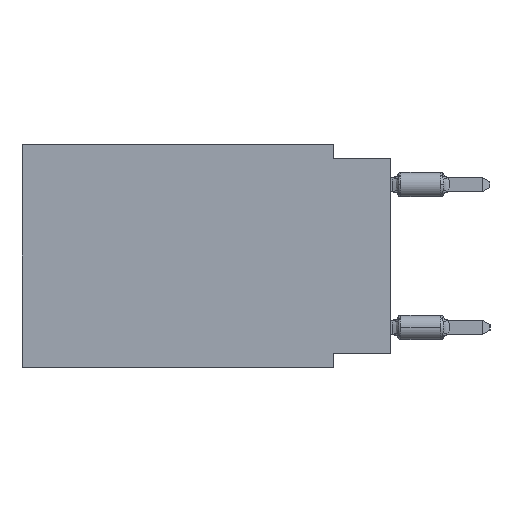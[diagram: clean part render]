
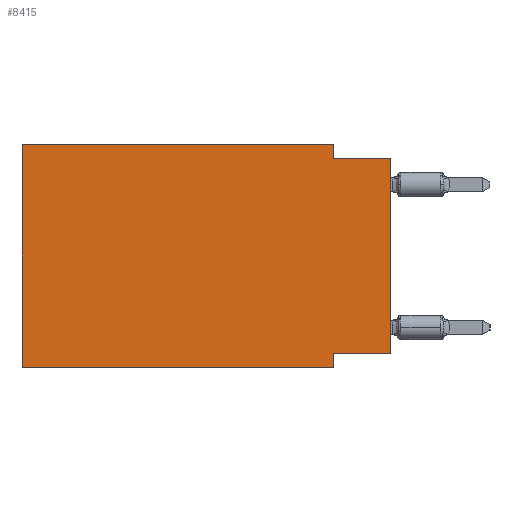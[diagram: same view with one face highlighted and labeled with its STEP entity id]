
A CAD part, left-side view. The second image highlights one B-rep face of the part: STEP entity #8415.
In plain terms, the highlighted planar face has unit normal (-1, 0, 0).
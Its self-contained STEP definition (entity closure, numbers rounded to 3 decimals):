
#71 = VECTOR ( 'NONE', #8384, 1000. ) ;
#573 = ORIENTED_EDGE ( 'NONE', *, *, #8297, .F. ) ;
#647 = VECTOR ( 'NONE', #6000, 1000. ) ;
#902 = VERTEX_POINT ( 'NONE', #19983 ) ;
#1110 = AXIS2_PLACEMENT_3D ( 'NONE', #20146, #5331, #11951 ) ;
#1647 = VERTEX_POINT ( 'NONE', #11638 ) ;
#1866 = CARTESIAN_POINT ( 'NONE',  ( 0., 2.54, -9.906 ) ) ;
#2638 = LINE ( 'NONE', #6296, #17011 ) ;
#3402 = PLANE ( 'NONE',  #1110 ) ;
#4509 = VERTEX_POINT ( 'NONE', #14054 ) ;
#4520 = LINE ( 'NONE', #7998, #15049 ) ;
#4533 = LINE ( 'NONE', #14067, #17102 ) ;
#5331 = DIRECTION ( 'NONE',  ( 1., 0., 0. ) ) ;
#5632 = VERTEX_POINT ( 'NONE', #18513 ) ;
#5681 = CARTESIAN_POINT ( 'NONE',  ( 0., 0., -0.635 ) ) ;
#5980 = DIRECTION ( 'NONE',  ( 0., 0., 1. ) ) ;
#6000 = DIRECTION ( 'NONE',  ( 0., 0., 1. ) ) ;
#6167 = CARTESIAN_POINT ( 'NONE',  ( 0., 2.54, 0. ) ) ;
#6296 = CARTESIAN_POINT ( 'NONE',  ( 0., 2.54, 0. ) ) ;
#6753 = FACE_OUTER_BOUND ( 'NONE', #12081, .T. ) ;
#7368 = DIRECTION ( 'NONE',  ( 0., -1., 0. ) ) ;
#7404 = ORIENTED_EDGE ( 'NONE', *, *, #13579, .F. ) ;
#7580 = DIRECTION ( 'NONE',  ( 0., -1., 0. ) ) ;
#7770 = VECTOR ( 'NONE', #7368, 1000. ) ;
#7865 = LINE ( 'NONE', #11325, #647 ) ;
#7998 = CARTESIAN_POINT ( 'NONE',  ( 0., 0., -9.271 ) ) ;
#8297 = EDGE_CURVE ( 'NONE', #1647, #11531, #18009, .T. ) ;
#8384 = DIRECTION ( 'NONE',  ( 0., -1., 0. ) ) ;
#8415 = ADVANCED_FACE ( 'NONE', ( #6753 ), #3402, .F. ) ;
#8666 = ORIENTED_EDGE ( 'NONE', *, *, #11497, .T. ) ;
#8861 = ORIENTED_EDGE ( 'NONE', *, *, #14319, .F. ) ;
#9248 = DIRECTION ( 'NONE',  ( 0., 0., -1. ) ) ;
#9490 = LINE ( 'NONE', #19407, #16055 ) ;
#10048 = CARTESIAN_POINT ( 'NONE',  ( 0., 0., -9.271 ) ) ;
#10129 = ORIENTED_EDGE ( 'NONE', *, *, #13762, .F. ) ;
#10167 = EDGE_CURVE ( 'NONE', #902, #1647, #17669, .T. ) ;
#11084 = CARTESIAN_POINT ( 'NONE',  ( 0., 16.383, 0. ) ) ;
#11325 = CARTESIAN_POINT ( 'NONE',  ( 0., 0., 0. ) ) ;
#11497 = EDGE_CURVE ( 'NONE', #902, #17876, #4533, .T. ) ;
#11531 = VERTEX_POINT ( 'NONE', #6167 ) ;
#11638 = CARTESIAN_POINT ( 'NONE',  ( 0., 16.383, 0. ) ) ;
#11951 = DIRECTION ( 'NONE',  ( 0., 0., -1. ) ) ;
#12081 = EDGE_LOOP ( 'NONE', ( #17341, #10129, #13791, #573, #13975, #8666, #7404, #8861 ) ) ;
#12350 = LINE ( 'NONE', #15488, #7770 ) ;
#12540 = VECTOR ( 'NONE', #5980, 1000. ) ;
#13579 = EDGE_CURVE ( 'NONE', #5632, #17876, #9490, .T. ) ;
#13762 = EDGE_CURVE ( 'NONE', #4509, #19685, #12350, .T. ) ;
#13791 = ORIENTED_EDGE ( 'NONE', *, *, #20259, .F. ) ;
#13975 = ORIENTED_EDGE ( 'NONE', *, *, #10167, .F. ) ;
#14054 = CARTESIAN_POINT ( 'NONE',  ( 0., 2.54, -0.635 ) ) ;
#14067 = CARTESIAN_POINT ( 'NONE',  ( 0., 16.383, -9.906 ) ) ;
#14319 = EDGE_CURVE ( 'NONE', #14513, #5632, #4520, .T. ) ;
#14513 = VERTEX_POINT ( 'NONE', #10048 ) ;
#15049 = VECTOR ( 'NONE', #19231, 1000. ) ;
#15488 = CARTESIAN_POINT ( 'NONE',  ( 0., 0., -0.635 ) ) ;
#16055 = VECTOR ( 'NONE', #20802, 1000. ) ;
#16391 = CARTESIAN_POINT ( 'NONE',  ( 0., 16.383, 0. ) ) ;
#17011 = VECTOR ( 'NONE', #9248, 1000. ) ;
#17102 = VECTOR ( 'NONE', #7580, 1000. ) ;
#17341 = ORIENTED_EDGE ( 'NONE', *, *, #18607, .T. ) ;
#17669 = LINE ( 'NONE', #11084, #12540 ) ;
#17876 = VERTEX_POINT ( 'NONE', #1866 ) ;
#18009 = LINE ( 'NONE', #16391, #71 ) ;
#18513 = CARTESIAN_POINT ( 'NONE',  ( 0., 2.54, -9.271 ) ) ;
#18607 = EDGE_CURVE ( 'NONE', #14513, #19685, #7865, .T. ) ;
#19231 = DIRECTION ( 'NONE',  ( 0., 1., 0. ) ) ;
#19407 = CARTESIAN_POINT ( 'NONE',  ( 0., 2.54, -9.906 ) ) ;
#19685 = VERTEX_POINT ( 'NONE', #5681 ) ;
#19983 = CARTESIAN_POINT ( 'NONE',  ( 0., 16.383, -9.906 ) ) ;
#20146 = CARTESIAN_POINT ( 'NONE',  ( 0., 16.383, 0. ) ) ;
#20259 = EDGE_CURVE ( 'NONE', #11531, #4509, #2638, .T. ) ;
#20802 = DIRECTION ( 'NONE',  ( 0., 0., -1. ) ) ;
